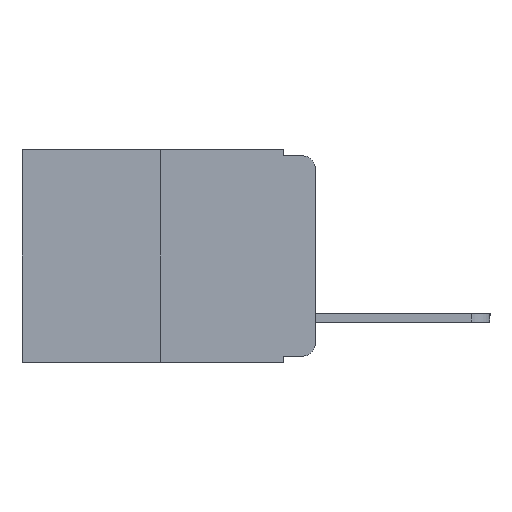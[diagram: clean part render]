
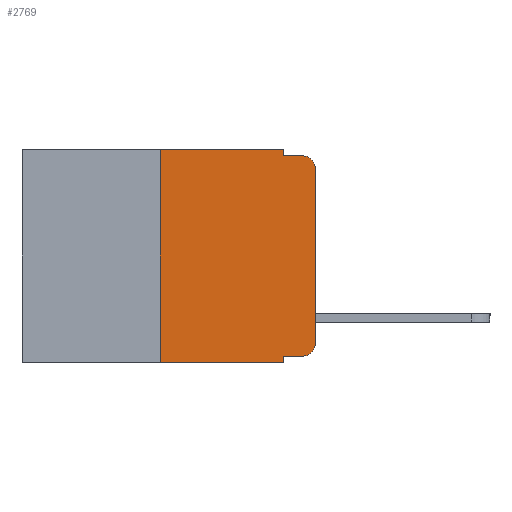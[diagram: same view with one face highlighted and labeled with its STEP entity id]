
A CAD part, left-side view. The second image highlights one B-rep face of the part: STEP entity #2769.
In plain terms, the highlighted planar face has unit normal (-1, 0, 0).
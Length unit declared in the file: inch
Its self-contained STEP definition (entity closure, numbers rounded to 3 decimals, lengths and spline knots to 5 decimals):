
#125 = LINE ( 'NONE', #5946, #14946 ) ;
#254 = VECTOR ( 'NONE', #12370, 39.37008 ) ;
#373 = EDGE_CURVE ( 'NONE', #18595, #11675, #23373, .T. ) ;
#689 = VERTEX_POINT ( 'NONE', #11391 ) ;
#995 = VERTEX_POINT ( 'NONE', #6591 ) ;
#1227 = ORIENTED_EDGE ( 'NONE', *, *, #12808, .F. ) ;
#1914 = EDGE_CURVE ( 'NONE', #17372, #995, #20132, .T. ) ;
#2131 = ORIENTED_EDGE ( 'NONE', *, *, #16889, .T. ) ;
#2237 = DIRECTION ( 'NONE',  ( 0., -1., 0. ) ) ;
#2290 = PLANE ( 'NONE',  #15068 ) ;
#2328 = CARTESIAN_POINT ( 'NONE',  ( 0., 0.473, 0. ) ) ;
#2387 = DIRECTION ( 'NONE',  ( 1., 0., 0. ) ) ;
#2464 = ORIENTED_EDGE ( 'NONE', *, *, #12079, .T. ) ;
#2769 = ADVANCED_FACE ( 'NONE', ( #19290 ), #2290, .F. ) ;
#2772 = DIRECTION ( 'NONE',  ( -1., 0., 0. ) ) ;
#3006 = ORIENTED_EDGE ( 'NONE', *, *, #4039, .T. ) ;
#3321 = EDGE_CURVE ( 'NONE', #19857, #995, #20764, .T. ) ;
#4039 = EDGE_CURVE ( 'NONE', #18651, #18844, #14879, .T. ) ;
#4313 = CARTESIAN_POINT ( 'NONE',  ( 0., 0.051, -0.333 ) ) ;
#5504 = EDGE_CURVE ( 'NONE', #689, #19857, #7365, .T. ) ;
#5946 = CARTESIAN_POINT ( 'NONE',  ( 0., 0.051, -0.333 ) ) ;
#6107 = VECTOR ( 'NONE', #9594, 39.37008 ) ;
#6164 = DIRECTION ( 'NONE',  ( 0., 0., -1. ) ) ;
#6510 = LINE ( 'NONE', #21801, #19124 ) ;
#6591 = CARTESIAN_POINT ( 'NONE',  ( 0., 0.02, -0.01 ) ) ;
#7365 = LINE ( 'NONE', #13200, #6107 ) ;
#7496 = EDGE_CURVE ( 'NONE', #11675, #17372, #6510, .T. ) ;
#7629 = AXIS2_PLACEMENT_3D ( 'NONE', #14077, #2772, #15861 ) ;
#8305 = CARTESIAN_POINT ( 'NONE',  ( 0., 0.25, 0. ) ) ;
#8729 = DIRECTION ( 'NONE',  ( -1., 0., 0. ) ) ;
#9136 = VECTOR ( 'NONE', #6164, 39.37008 ) ;
#9355 = CARTESIAN_POINT ( 'NONE',  ( 0., 0.051, -0.01 ) ) ;
#9594 = DIRECTION ( 'NONE',  ( 0., 0., 1. ) ) ;
#9656 = AXIS2_PLACEMENT_3D ( 'NONE', #19276, #8729, #20895 ) ;
#9726 = DIRECTION ( 'NONE',  ( 0., 0., -1. ) ) ;
#10543 = CIRCLE ( 'NONE', #9656, 0.02 ) ;
#10572 = CARTESIAN_POINT ( 'NONE',  ( 0., 0.25, 0. ) ) ;
#10662 = CARTESIAN_POINT ( 'NONE',  ( 0., 0., -0.03 ) ) ;
#11167 = EDGE_LOOP ( 'NONE', ( #15764, #15730, #16508, #15059, #15294, #16620, #3006, #1227, #2131, #2464 ) ) ;
#11234 = CARTESIAN_POINT ( 'NONE',  ( 0., 0.473, -0.343 ) ) ;
#11391 = CARTESIAN_POINT ( 'NONE',  ( 0., 0., -0.313 ) ) ;
#11675 = VERTEX_POINT ( 'NONE', #15280 ) ;
#12079 = EDGE_CURVE ( 'NONE', #19565, #689, #10543, .T. ) ;
#12370 = DIRECTION ( 'NONE',  ( 0., 0., 1. ) ) ;
#12808 = EDGE_CURVE ( 'NONE', #18561, #18844, #13915, .T. ) ;
#12985 = DIRECTION ( 'NONE',  ( 0., -1., 0. ) ) ;
#13200 = CARTESIAN_POINT ( 'NONE',  ( 0., 0., 0. ) ) ;
#13529 = CARTESIAN_POINT ( 'NONE',  ( 0., 0.051, -0.01 ) ) ;
#13915 = LINE ( 'NONE', #17124, #9136 ) ;
#14077 = CARTESIAN_POINT ( 'NONE',  ( 0., 0.02, -0.03 ) ) ;
#14879 = LINE ( 'NONE', #11234, #22246 ) ;
#14946 = VECTOR ( 'NONE', #23464, 39.37008 ) ;
#15059 = ORIENTED_EDGE ( 'NONE', *, *, #7496, .F. ) ;
#15068 = AXIS2_PLACEMENT_3D ( 'NONE', #18915, #2387, #15568 ) ;
#15122 = VECTOR ( 'NONE', #15377, 39.37008 ) ;
#15280 = CARTESIAN_POINT ( 'NONE',  ( 0., 0.051, 0. ) ) ;
#15294 = ORIENTED_EDGE ( 'NONE', *, *, #373, .F. ) ;
#15377 = DIRECTION ( 'NONE',  ( 0., -1., 0. ) ) ;
#15568 = DIRECTION ( 'NONE',  ( 0., 0., -1. ) ) ;
#15619 = LINE ( 'NONE', #10572, #254 ) ;
#15730 = ORIENTED_EDGE ( 'NONE', *, *, #3321, .T. ) ;
#15764 = ORIENTED_EDGE ( 'NONE', *, *, #5504, .T. ) ;
#15861 = DIRECTION ( 'NONE',  ( 0., 0., -1. ) ) ;
#16508 = ORIENTED_EDGE ( 'NONE', *, *, #1914, .F. ) ;
#16620 = ORIENTED_EDGE ( 'NONE', *, *, #19774, .F. ) ;
#16889 = EDGE_CURVE ( 'NONE', #18561, #19565, #125, .T. ) ;
#17124 = CARTESIAN_POINT ( 'NONE',  ( 0., 0.051, 0. ) ) ;
#17372 = VERTEX_POINT ( 'NONE', #9355 ) ;
#17374 = CARTESIAN_POINT ( 'NONE',  ( 0., 0.02, -0.333 ) ) ;
#17399 = CARTESIAN_POINT ( 'NONE',  ( 0., 0.25, -0.343 ) ) ;
#18561 = VERTEX_POINT ( 'NONE', #4313 ) ;
#18595 = VERTEX_POINT ( 'NONE', #8305 ) ;
#18651 = VERTEX_POINT ( 'NONE', #17399 ) ;
#18844 = VERTEX_POINT ( 'NONE', #22631 ) ;
#18915 = CARTESIAN_POINT ( 'NONE',  ( 0., 0.473, 0. ) ) ;
#18995 = VECTOR ( 'NONE', #2237, 39.37008 ) ;
#19124 = VECTOR ( 'NONE', #9726, 39.37008 ) ;
#19276 = CARTESIAN_POINT ( 'NONE',  ( 0., 0.02, -0.313 ) ) ;
#19290 = FACE_OUTER_BOUND ( 'NONE', #11167, .T. ) ;
#19565 = VERTEX_POINT ( 'NONE', #17374 ) ;
#19774 = EDGE_CURVE ( 'NONE', #18651, #18595, #15619, .T. ) ;
#19857 = VERTEX_POINT ( 'NONE', #10662 ) ;
#20132 = LINE ( 'NONE', #13529, #15122 ) ;
#20764 = CIRCLE ( 'NONE', #7629, 0.02 ) ;
#20895 = DIRECTION ( 'NONE',  ( 0., 0., -1. ) ) ;
#21801 = CARTESIAN_POINT ( 'NONE',  ( 0., 0.051, 0. ) ) ;
#22246 = VECTOR ( 'NONE', #12985, 39.37008 ) ;
#22631 = CARTESIAN_POINT ( 'NONE',  ( 0., 0.051, -0.343 ) ) ;
#23373 = LINE ( 'NONE', #2328, #18995 ) ;
#23464 = DIRECTION ( 'NONE',  ( 0., -1., 0. ) ) ;
